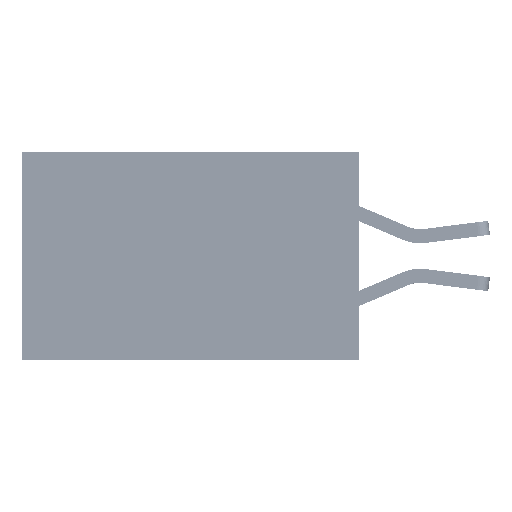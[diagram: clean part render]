
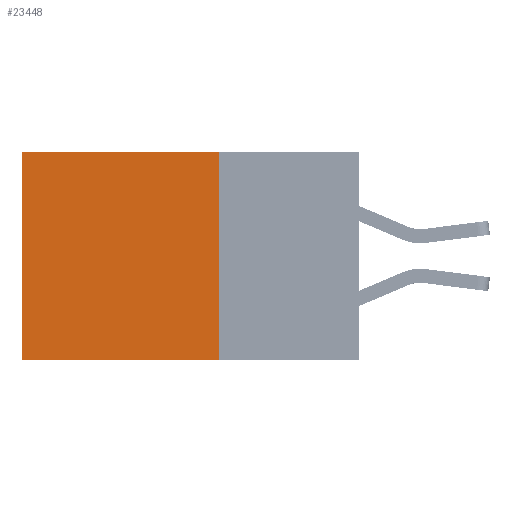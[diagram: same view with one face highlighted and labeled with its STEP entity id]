
A CAD part, left-side view. The second image highlights one B-rep face of the part: STEP entity #23448.
In plain terms, the highlighted planar face has unit normal (-1, 0, 0).
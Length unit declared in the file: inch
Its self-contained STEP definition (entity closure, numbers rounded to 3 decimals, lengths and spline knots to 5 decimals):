
#301 = CARTESIAN_POINT ( 'NONE',  ( 0.2875, 0.25, 0. ) ) ;
#2635 = CARTESIAN_POINT ( 'NONE',  ( 0.2875, 0.6, -0.37 ) ) ;
#3493 = EDGE_CURVE ( 'NONE', #3533, #35116, #23916, .T. ) ;
#3533 = VERTEX_POINT ( 'NONE', #4104 ) ;
#3590 = EDGE_LOOP ( 'NONE', ( #19297, #27443, #15868, #5554 ) ) ;
#4104 = CARTESIAN_POINT ( 'NONE',  ( 0.2875, 0.25, 0. ) ) ;
#4936 = VERTEX_POINT ( 'NONE', #2635 ) ;
#5554 = ORIENTED_EDGE ( 'NONE', *, *, #3493, .T. ) ;
#7429 = VECTOR ( 'NONE', #12826, 39.37008 ) ;
#9547 = EDGE_CURVE ( 'NONE', #22001, #4936, #38747, .T. ) ;
#9791 = CARTESIAN_POINT ( 'NONE',  ( 0.2875, 0.25, 0. ) ) ;
#11400 = CARTESIAN_POINT ( 'NONE',  ( 0.2875, 0.6, 0. ) ) ;
#11886 = EDGE_CURVE ( 'NONE', #35116, #4936, #12483, .T. ) ;
#12000 = CARTESIAN_POINT ( 'NONE',  ( 0.2875, 0.25, -0.37 ) ) ;
#12467 = CARTESIAN_POINT ( 'NONE',  ( 0.2875, 0.6, 0. ) ) ;
#12483 = LINE ( 'NONE', #11400, #32838 ) ;
#12599 = PLANE ( 'NONE',  #19277 ) ;
#12826 = DIRECTION ( 'NONE',  ( 0., 0., -1. ) ) ;
#12956 = DIRECTION ( 'NONE',  ( 0., 1., 0. ) ) ;
#13811 = CARTESIAN_POINT ( 'NONE',  ( 0.2875, 0.25, -0.37 ) ) ;
#15868 = ORIENTED_EDGE ( 'NONE', *, *, #37700, .F. ) ;
#19018 = FACE_OUTER_BOUND ( 'NONE', #3590, .T. ) ;
#19277 = AXIS2_PLACEMENT_3D ( 'NONE', #23178, #25672, #32050 ) ;
#19297 = ORIENTED_EDGE ( 'NONE', *, *, #11886, .T. ) ;
#20525 = DIRECTION ( 'NONE',  ( 0., 0., -1. ) ) ;
#22001 = VERTEX_POINT ( 'NONE', #13811 ) ;
#23178 = CARTESIAN_POINT ( 'NONE',  ( 0.2875, 0.25, 0. ) ) ;
#23448 = ADVANCED_FACE ( 'NONE', ( #19018 ), #12599, .F. ) ;
#23916 = LINE ( 'NONE', #9791, #31014 ) ;
#25482 = VECTOR ( 'NONE', #33416, 39.37008 ) ;
#25672 = DIRECTION ( 'NONE',  ( 1., 0., 0. ) ) ;
#27443 = ORIENTED_EDGE ( 'NONE', *, *, #9547, .F. ) ;
#30152 = LINE ( 'NONE', #301, #7429 ) ;
#31014 = VECTOR ( 'NONE', #12956, 39.37008 ) ;
#32050 = DIRECTION ( 'NONE',  ( 0., 0., -1. ) ) ;
#32838 = VECTOR ( 'NONE', #20525, 39.37008 ) ;
#33416 = DIRECTION ( 'NONE',  ( 0., 1., 0. ) ) ;
#35116 = VERTEX_POINT ( 'NONE', #12467 ) ;
#37700 = EDGE_CURVE ( 'NONE', #3533, #22001, #30152, .T. ) ;
#38747 = LINE ( 'NONE', #12000, #25482 ) ;
